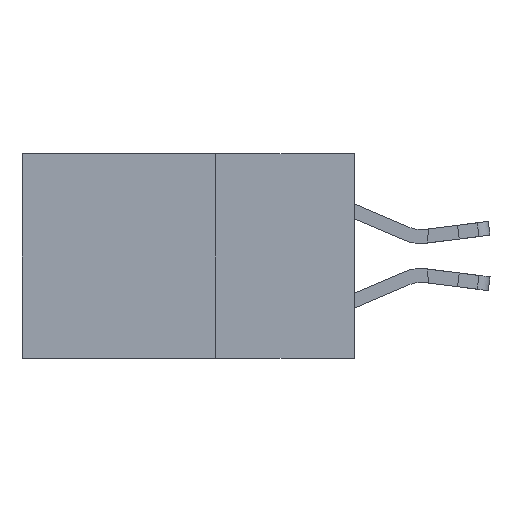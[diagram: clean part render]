
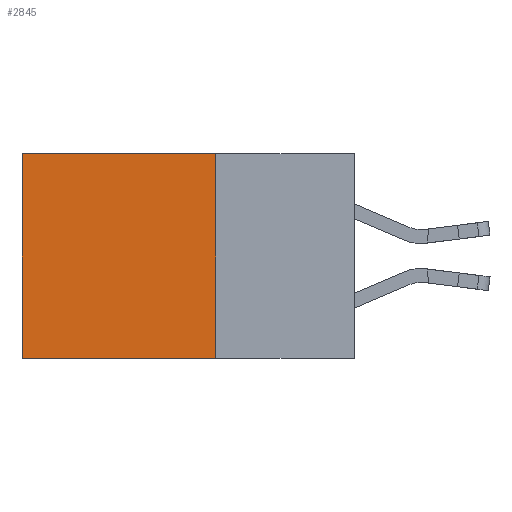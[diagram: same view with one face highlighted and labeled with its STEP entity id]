
A CAD part, left-side view. The second image highlights one B-rep face of the part: STEP entity #2845.
In plain terms, the highlighted planar face has unit normal (-1, 0, 0).
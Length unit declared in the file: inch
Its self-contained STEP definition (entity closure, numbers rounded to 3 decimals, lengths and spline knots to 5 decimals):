
#215 = VECTOR ( 'NONE', #10751, 39.37008 ) ;
#225 = VERTEX_POINT ( 'NONE', #11589 ) ;
#1086 = DIRECTION ( 'NONE',  ( 0., 0., -1. ) ) ;
#1544 = VECTOR ( 'NONE', #6689, 39.37008 ) ;
#1675 = CARTESIAN_POINT ( 'NONE',  ( 0.2615, 0.6, -0.37 ) ) ;
#1732 = VERTEX_POINT ( 'NONE', #8433 ) ;
#2350 = VECTOR ( 'NONE', #1086, 39.37008 ) ;
#2845 = ADVANCED_FACE ( 'NONE', ( #9329 ), #12455, .F. ) ;
#3043 = LINE ( 'NONE', #10745, #215 ) ;
#3568 = AXIS2_PLACEMENT_3D ( 'NONE', #12613, #12418, #12381 ) ;
#6432 = VERTEX_POINT ( 'NONE', #12587 ) ;
#6521 = CARTESIAN_POINT ( 'NONE',  ( 0.2615, 0.25, -0.37 ) ) ;
#6664 = VERTEX_POINT ( 'NONE', #11218 ) ;
#6689 = DIRECTION ( 'NONE',  ( 0., 0., -1. ) ) ;
#6721 = EDGE_CURVE ( 'NONE', #6432, #225, #3043, .T. ) ;
#7273 = EDGE_LOOP ( 'NONE', ( #8578, #9819, #9222, #9177 ) ) ;
#7800 = LINE ( 'NONE', #1675, #2350 ) ;
#8433 = CARTESIAN_POINT ( 'NONE',  ( 0.2615, 0.6, 0. ) ) ;
#8578 = ORIENTED_EDGE ( 'NONE', *, *, #12612, .T. ) ;
#9177 = ORIENTED_EDGE ( 'NONE', *, *, #13214, .T. ) ;
#9222 = ORIENTED_EDGE ( 'NONE', *, *, #12421, .F. ) ;
#9329 = FACE_OUTER_BOUND ( 'NONE', #7273, .T. ) ;
#9433 = DIRECTION ( 'NONE',  ( 0., 1., 0. ) ) ;
#9819 = ORIENTED_EDGE ( 'NONE', *, *, #6721, .F. ) ;
#9859 = CARTESIAN_POINT ( 'NONE',  ( 0.2615, 0.25, 0. ) ) ;
#10745 = CARTESIAN_POINT ( 'NONE',  ( 0.2615, 0.25, -0.37 ) ) ;
#10751 = DIRECTION ( 'NONE',  ( 0., 1., 0. ) ) ;
#11218 = CARTESIAN_POINT ( 'NONE',  ( 0.2615, 0.25, 0. ) ) ;
#11589 = CARTESIAN_POINT ( 'NONE',  ( 0.2615, 0.6, -0.37 ) ) ;
#12371 = VECTOR ( 'NONE', #9433, 39.37008 ) ;
#12381 = DIRECTION ( 'NONE',  ( 0., 0., -1. ) ) ;
#12418 = DIRECTION ( 'NONE',  ( 1., 0., 0. ) ) ;
#12421 = EDGE_CURVE ( 'NONE', #6664, #6432, #12698, .T. ) ;
#12455 = PLANE ( 'NONE',  #3568 ) ;
#12587 = CARTESIAN_POINT ( 'NONE',  ( 0.2615, 0.25, -0.37 ) ) ;
#12612 = EDGE_CURVE ( 'NONE', #1732, #225, #7800, .T. ) ;
#12613 = CARTESIAN_POINT ( 'NONE',  ( 0.2615, 0.25, -0.37 ) ) ;
#12678 = LINE ( 'NONE', #9859, #12371 ) ;
#12698 = LINE ( 'NONE', #6521, #1544 ) ;
#13214 = EDGE_CURVE ( 'NONE', #6664, #1732, #12678, .T. ) ;
